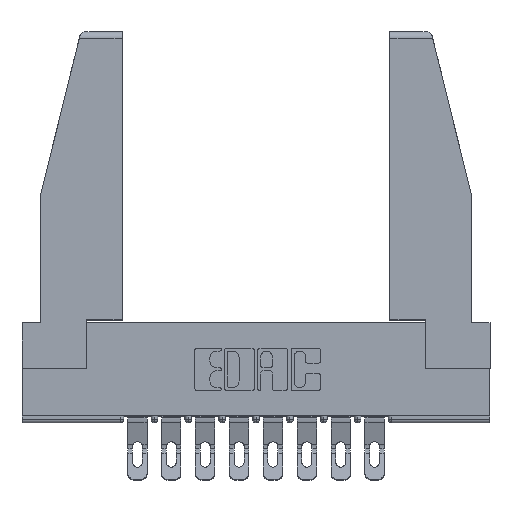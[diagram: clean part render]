
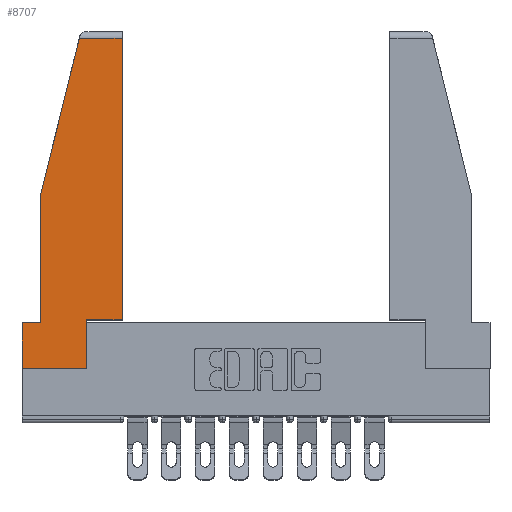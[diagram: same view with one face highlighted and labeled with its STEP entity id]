
A CAD part, top view. The second image highlights one B-rep face of the part: STEP entity #8707.
In plain terms, the highlighted planar face has unit normal (0, 0, 1).
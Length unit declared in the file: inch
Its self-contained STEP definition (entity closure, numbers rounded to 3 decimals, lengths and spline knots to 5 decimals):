
#329 = CARTESIAN_POINT ( 'NONE',  ( 0., 0., 0. ) ) ;
#344 = CARTESIAN_POINT ( 'NONE',  ( 0.297, 0., 0. ) ) ;
#937 = CARTESIAN_POINT ( 'NONE',  ( 0., 0.21, 0. ) ) ;
#1033 = PLANE ( 'NONE',  #2319 ) ;
#1073 = DIRECTION ( 'NONE',  ( -1., 0., 0. ) ) ;
#1511 = CARTESIAN_POINT ( 'NONE',  ( 0.297, 0.223, 0. ) ) ;
#1748 = LINE ( 'NONE', #4839, #7507 ) ;
#1807 = EDGE_LOOP ( 'NONE', ( #13190, #3075, #4328, #4265, #8762, #3908, #10210, #7949, #8219 ) ) ;
#2154 = CARTESIAN_POINT ( 'NONE',  ( 0.461, 1.52, 0. ) ) ;
#2319 = AXIS2_PLACEMENT_3D ( 'NONE', #9660, #3522, #12120 ) ;
#2614 = DIRECTION ( 'NONE',  ( 0., 1., 0. ) ) ;
#2785 = VERTEX_POINT ( 'NONE', #7916 ) ;
#2797 = LINE ( 'NONE', #5443, #11465 ) ;
#2880 = DIRECTION ( 'NONE',  ( 1., 0., 0. ) ) ;
#2972 = VECTOR ( 'NONE', #3582, 39.37008 ) ;
#3075 = ORIENTED_EDGE ( 'NONE', *, *, #6647, .T. ) ;
#3522 = DIRECTION ( 'NONE',  ( 0., 0., 1. ) ) ;
#3582 = DIRECTION ( 'NONE',  ( 0., -1., 0. ) ) ;
#3908 = ORIENTED_EDGE ( 'NONE', *, *, #6903, .T. ) ;
#4064 = DIRECTION ( 'NONE',  ( 0., 1., 0. ) ) ;
#4156 = VERTEX_POINT ( 'NONE', #329 ) ;
#4211 = LINE ( 'NONE', #12478, #10599 ) ;
#4265 = ORIENTED_EDGE ( 'NONE', *, *, #10296, .T. ) ;
#4328 = ORIENTED_EDGE ( 'NONE', *, *, #15116, .T. ) ;
#4462 = LINE ( 'NONE', #5048, #9091 ) ;
#4839 = CARTESIAN_POINT ( 'NONE',  ( 0., 0.21, 0. ) ) ;
#5048 = CARTESIAN_POINT ( 'NONE',  ( 0.461, 0.223, 0. ) ) ;
#5315 = DIRECTION ( 'NONE',  ( -1., 0., 0. ) ) ;
#5389 = VECTOR ( 'NONE', #2880, 39.37008 ) ;
#5443 = CARTESIAN_POINT ( 'NONE',  ( 0.297, 0.223, 0. ) ) ;
#5734 = EDGE_CURVE ( 'NONE', #12573, #10696, #2797, .T. ) ;
#5853 = VERTEX_POINT ( 'NONE', #6699 ) ;
#6647 = EDGE_CURVE ( 'NONE', #11186, #14398, #10708, .T. ) ;
#6654 = CARTESIAN_POINT ( 'NONE',  ( 0., 1.52, 0. ) ) ;
#6699 = CARTESIAN_POINT ( 'NONE',  ( 0.297, 0., 0. ) ) ;
#6703 = CARTESIAN_POINT ( 'NONE',  ( 0.461, 0.223, 0. ) ) ;
#6729 = FACE_OUTER_BOUND ( 'NONE', #1807, .T. ) ;
#6903 = EDGE_CURVE ( 'NONE', #10248, #4156, #15235, .T. ) ;
#7299 = DIRECTION ( 'NONE',  ( -0.239, -0.971, 0. ) ) ;
#7507 = VECTOR ( 'NONE', #1073, 39.37008 ) ;
#7645 = CARTESIAN_POINT ( 'NONE',  ( 0., 0., 0. ) ) ;
#7916 = CARTESIAN_POINT ( 'NONE',  ( 0.086, 0.21, 0. ) ) ;
#7949 = ORIENTED_EDGE ( 'NONE', *, *, #9915, .T. ) ;
#8219 = ORIENTED_EDGE ( 'NONE', *, *, #5734, .T. ) ;
#8676 = CARTESIAN_POINT ( 'NONE',  ( 0., 0.21, 0. ) ) ;
#8707 = ADVANCED_FACE ( 'NONE', ( #6729 ), #1033, .T. ) ;
#8750 = VECTOR ( 'NONE', #5315, 39.37008 ) ;
#8762 = ORIENTED_EDGE ( 'NONE', *, *, #15120, .T. ) ;
#8950 = EDGE_CURVE ( 'NONE', #4156, #5853, #9263, .T. ) ;
#9091 = VECTOR ( 'NONE', #2614, 39.37008 ) ;
#9263 = LINE ( 'NONE', #7645, #5389 ) ;
#9505 = DIRECTION ( 'NONE',  ( 1., 0., 0. ) ) ;
#9660 = CARTESIAN_POINT ( 'NONE',  ( 0., 0., 0. ) ) ;
#9915 = EDGE_CURVE ( 'NONE', #5853, #12573, #13627, .T. ) ;
#9933 = DIRECTION ( 'NONE',  ( 0., -1., 0. ) ) ;
#10083 = CARTESIAN_POINT ( 'NONE',  ( 0.2636, 1.52, 0. ) ) ;
#10210 = ORIENTED_EDGE ( 'NONE', *, *, #8950, .T. ) ;
#10248 = VERTEX_POINT ( 'NONE', #8676 ) ;
#10296 = EDGE_CURVE ( 'NONE', #10652, #2785, #4211, .T. ) ;
#10599 = VECTOR ( 'NONE', #9933, 39.37008 ) ;
#10645 = LINE ( 'NONE', #13488, #15192 ) ;
#10652 = VERTEX_POINT ( 'NONE', #15469 ) ;
#10696 = VERTEX_POINT ( 'NONE', #6703 ) ;
#10708 = LINE ( 'NONE', #6654, #8750 ) ;
#11186 = VERTEX_POINT ( 'NONE', #2154 ) ;
#11465 = VECTOR ( 'NONE', #9505, 39.37008 ) ;
#12120 = DIRECTION ( 'NONE',  ( 1., 0., 0. ) ) ;
#12478 = CARTESIAN_POINT ( 'NONE',  ( 0.086, 0.8, 0. ) ) ;
#12573 = VERTEX_POINT ( 'NONE', #1511 ) ;
#13190 = ORIENTED_EDGE ( 'NONE', *, *, #15266, .T. ) ;
#13264 = VECTOR ( 'NONE', #4064, 39.37008 ) ;
#13488 = CARTESIAN_POINT ( 'NONE',  ( 0.271, 1.55, 0. ) ) ;
#13627 = LINE ( 'NONE', #344, #13264 ) ;
#14398 = VERTEX_POINT ( 'NONE', #10083 ) ;
#15116 = EDGE_CURVE ( 'NONE', #14398, #10652, #10645, .T. ) ;
#15120 = EDGE_CURVE ( 'NONE', #2785, #10248, #1748, .T. ) ;
#15192 = VECTOR ( 'NONE', #7299, 39.37008 ) ;
#15235 = LINE ( 'NONE', #937, #2972 ) ;
#15266 = EDGE_CURVE ( 'NONE', #10696, #11186, #4462, .T. ) ;
#15469 = CARTESIAN_POINT ( 'NONE',  ( 0.086, 0.8, 0. ) ) ;
